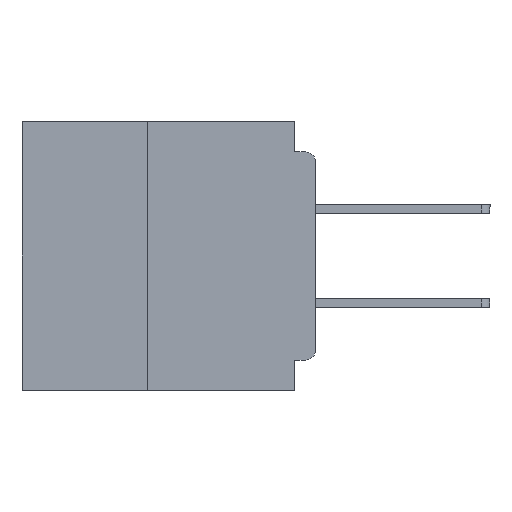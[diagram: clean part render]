
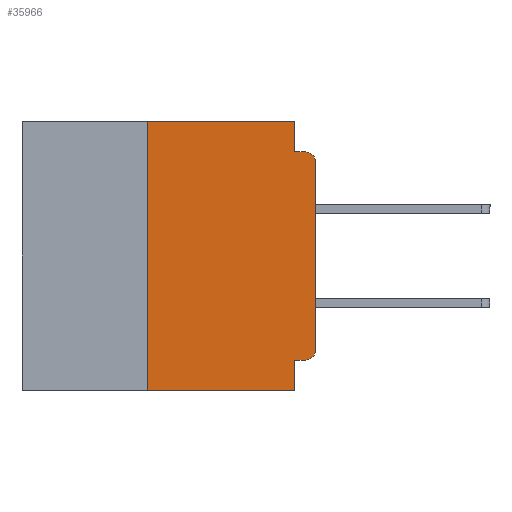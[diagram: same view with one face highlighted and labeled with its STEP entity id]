
A CAD part, left-side view. The second image highlights one B-rep face of the part: STEP entity #35966.
In plain terms, the highlighted planar face has unit normal (-1, 0, 0).
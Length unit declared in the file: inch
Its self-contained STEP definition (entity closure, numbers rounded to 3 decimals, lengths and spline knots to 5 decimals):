
#248 = EDGE_CURVE ( 'NONE', #43087, #16383, #6548, .T. ) ;
#633 = VECTOR ( 'NONE', #44646, 39.37008 ) ;
#1960 = DIRECTION ( 'NONE',  ( 0., 0., 1. ) ) ;
#2380 = CARTESIAN_POINT ( 'NONE',  ( 0., 0.437, 0. ) ) ;
#2517 = LINE ( 'NONE', #13548, #40561 ) ;
#2589 = FACE_OUTER_BOUND ( 'NONE', #45895, .T. ) ;
#2665 = VECTOR ( 'NONE', #16168, 39.37008 ) ;
#2679 = PLANE ( 'NONE',  #44750 ) ;
#3781 = CARTESIAN_POINT ( 'NONE',  ( 0., 0.031, -0.355 ) ) ;
#4283 = DIRECTION ( 'NONE',  ( -1., 0., 0. ) ) ;
#4506 = CARTESIAN_POINT ( 'NONE',  ( 0., 0., -0.06 ) ) ;
#5024 = CARTESIAN_POINT ( 'NONE',  ( 0., 0.015, -0.355 ) ) ;
#5344 = EDGE_CURVE ( 'NONE', #11714, #30849, #37844, .T. ) ;
#5664 = VECTOR ( 'NONE', #18934, 39.37008 ) ;
#6072 = CARTESIAN_POINT ( 'NONE',  ( 0., 0.031, -0.045 ) ) ;
#6134 = VERTEX_POINT ( 'NONE', #33630 ) ;
#6548 = LINE ( 'NONE', #33238, #33668 ) ;
#7435 = VERTEX_POINT ( 'NONE', #5024 ) ;
#7786 = VECTOR ( 'NONE', #26845, 39.37008 ) ;
#8580 = EDGE_CURVE ( 'NONE', #30012, #16383, #17137, .T. ) ;
#8766 = DIRECTION ( 'NONE',  ( -1., 0., 0. ) ) ;
#10101 = DIRECTION ( 'NONE',  ( 0., 0., -1. ) ) ;
#10446 = LINE ( 'NONE', #18928, #633 ) ;
#11669 = ORIENTED_EDGE ( 'NONE', *, *, #22478, .T. ) ;
#11714 = VERTEX_POINT ( 'NONE', #13839 ) ;
#13408 = ORIENTED_EDGE ( 'NONE', *, *, #31373, .F. ) ;
#13548 = CARTESIAN_POINT ( 'NONE',  ( 0., 0.031, 0. ) ) ;
#13839 = CARTESIAN_POINT ( 'NONE',  ( 0., 0.25, 0. ) ) ;
#15889 = AXIS2_PLACEMENT_3D ( 'NONE', #26319, #4283, #30020 ) ;
#16168 = DIRECTION ( 'NONE',  ( 0., 1., 0. ) ) ;
#16302 = ORIENTED_EDGE ( 'NONE', *, *, #25859, .F. ) ;
#16383 = VERTEX_POINT ( 'NONE', #46076 ) ;
#16774 = VECTOR ( 'NONE', #1960, 39.37008 ) ;
#17038 = VECTOR ( 'NONE', #24414, 39.37008 ) ;
#17137 = CIRCLE ( 'NONE', #15889, 0.015 ) ;
#17552 = LINE ( 'NONE', #45171, #7786 ) ;
#17925 = LINE ( 'NONE', #46043, #16774 ) ;
#18928 = CARTESIAN_POINT ( 'NONE',  ( 0., 0., 0. ) ) ;
#18934 = DIRECTION ( 'NONE',  ( 0., 0., -1. ) ) ;
#21160 = CARTESIAN_POINT ( 'NONE',  ( 0., 0.031, 0. ) ) ;
#22478 = EDGE_CURVE ( 'NONE', #6134, #30012, #10446, .T. ) ;
#23955 = EDGE_CURVE ( 'NONE', #32638, #41437, #24108, .T. ) ;
#24108 = LINE ( 'NONE', #41008, #5664 ) ;
#24337 = ORIENTED_EDGE ( 'NONE', *, *, #26429, .T. ) ;
#24414 = DIRECTION ( 'NONE',  ( 0., -1., 0. ) ) ;
#24622 = DIRECTION ( 'NONE',  ( 0., 0., -1. ) ) ;
#25859 = EDGE_CURVE ( 'NONE', #7435, #32638, #30913, .T. ) ;
#26319 = CARTESIAN_POINT ( 'NONE',  ( 0., 0.015, -0.06 ) ) ;
#26429 = EDGE_CURVE ( 'NONE', #38655, #41437, #17552, .T. ) ;
#26845 = DIRECTION ( 'NONE',  ( 0., -1., 0. ) ) ;
#28367 = ORIENTED_EDGE ( 'NONE', *, *, #38816, .F. ) ;
#28923 = CARTESIAN_POINT ( 'NONE',  ( 0., 0.031, -0.4 ) ) ;
#29593 = ORIENTED_EDGE ( 'NONE', *, *, #46469, .T. ) ;
#30012 = VERTEX_POINT ( 'NONE', #4506 ) ;
#30020 = DIRECTION ( 'NONE',  ( 0., 0., -1. ) ) ;
#30835 = CARTESIAN_POINT ( 'NONE',  ( 0., 0.015, -0.34 ) ) ;
#30849 = VERTEX_POINT ( 'NONE', #21160 ) ;
#30913 = LINE ( 'NONE', #38285, #2665 ) ;
#31256 = ORIENTED_EDGE ( 'NONE', *, *, #8580, .T. ) ;
#31373 = EDGE_CURVE ( 'NONE', #38655, #11714, #17925, .T. ) ;
#32143 = DIRECTION ( 'NONE',  ( 1., 0., 0. ) ) ;
#32638 = VERTEX_POINT ( 'NONE', #3781 ) ;
#33229 = DIRECTION ( 'NONE',  ( 0., -1., 0. ) ) ;
#33238 = CARTESIAN_POINT ( 'NONE',  ( 0., 0., -0.045 ) ) ;
#33579 = ORIENTED_EDGE ( 'NONE', *, *, #248, .F. ) ;
#33630 = CARTESIAN_POINT ( 'NONE',  ( 0., 0., -0.34 ) ) ;
#33668 = VECTOR ( 'NONE', #33229, 39.37008 ) ;
#34531 = DIRECTION ( 'NONE',  ( 0., 0., -1. ) ) ;
#35375 = CIRCLE ( 'NONE', #42940, 0.015 ) ;
#35966 = ADVANCED_FACE ( 'NONE', ( #2589 ), #2679, .F. ) ;
#37844 = LINE ( 'NONE', #2380, #17038 ) ;
#38285 = CARTESIAN_POINT ( 'NONE',  ( 0., 0., -0.355 ) ) ;
#38392 = CARTESIAN_POINT ( 'NONE',  ( 0., 0.25, -0.4 ) ) ;
#38655 = VERTEX_POINT ( 'NONE', #38392 ) ;
#38816 = EDGE_CURVE ( 'NONE', #30849, #43087, #2517, .T. ) ;
#39359 = ORIENTED_EDGE ( 'NONE', *, *, #5344, .F. ) ;
#40561 = VECTOR ( 'NONE', #24622, 39.37008 ) ;
#41008 = CARTESIAN_POINT ( 'NONE',  ( 0., 0.031, -0.4 ) ) ;
#41094 = ORIENTED_EDGE ( 'NONE', *, *, #23955, .F. ) ;
#41437 = VERTEX_POINT ( 'NONE', #28923 ) ;
#42940 = AXIS2_PLACEMENT_3D ( 'NONE', #30835, #8766, #34531 ) ;
#43067 = CARTESIAN_POINT ( 'NONE',  ( 0., 0.437, 0. ) ) ;
#43087 = VERTEX_POINT ( 'NONE', #6072 ) ;
#44646 = DIRECTION ( 'NONE',  ( 0., 0., 1. ) ) ;
#44750 = AXIS2_PLACEMENT_3D ( 'NONE', #43067, #32143, #10101 ) ;
#45171 = CARTESIAN_POINT ( 'NONE',  ( 0., 0.437, -0.4 ) ) ;
#45895 = EDGE_LOOP ( 'NONE', ( #11669, #31256, #33579, #28367, #39359, #13408, #24337, #41094, #16302, #29593 ) ) ;
#46043 = CARTESIAN_POINT ( 'NONE',  ( 0., 0.25, -0.4 ) ) ;
#46076 = CARTESIAN_POINT ( 'NONE',  ( 0., 0.015, -0.045 ) ) ;
#46469 = EDGE_CURVE ( 'NONE', #7435, #6134, #35375, .T. ) ;
